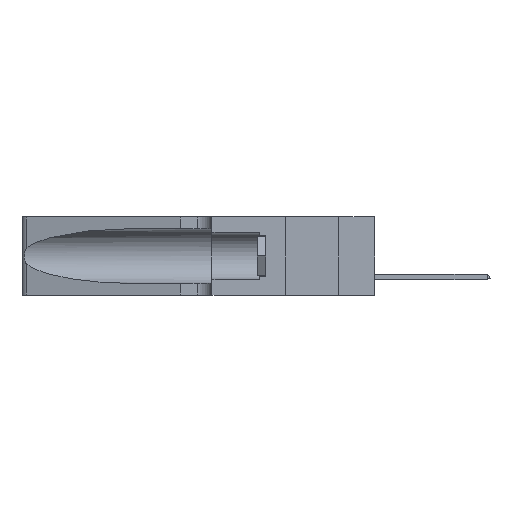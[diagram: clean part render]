
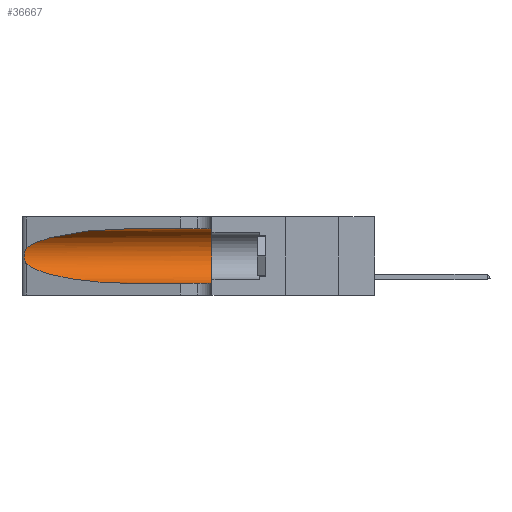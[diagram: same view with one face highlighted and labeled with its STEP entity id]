
A CAD part, left-side view. The second image highlights one B-rep face of the part: STEP entity #36667.
In plain terms, the highlighted cylindrical face has radius 3.308 mm (diameter 6.617 mm), a partial arc.
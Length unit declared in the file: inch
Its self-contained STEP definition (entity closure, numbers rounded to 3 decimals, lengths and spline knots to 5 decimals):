
#444 = CARTESIAN_POINT ( 'NONE',  ( 0.18966, 0.96281, 0.05475 ) ) ;
#1295 = LINE ( 'NONE', #36476, #23043 ) ;
#1427 = CYLINDRICAL_SURFACE ( 'NONE', #3161, 0.13025 ) ;
#3161 = AXIS2_PLACEMENT_3D ( 'NONE', #37629, #3948, #16302 ) ;
#3672 = ORIENTED_EDGE ( 'NONE', *, *, #19478, .F. ) ;
#3948 = DIRECTION ( 'NONE',  ( 0., -1., 0. ) ) ;
#4481 = CARTESIAN_POINT ( 'NONE',  ( 0.1305, 0.35, 0.31525 ) ) ;
#4510 = ORIENTED_EDGE ( 'NONE', *, *, #5658, .T. ) ;
#4600 = EDGE_CURVE ( 'NONE', #29638, #32882, #22584, .T. ) ;
#5658 = EDGE_CURVE ( 'NONE', #21468, #32882, #39531, .T. ) ;
#6064 = ORIENTED_EDGE ( 'NONE', *, *, #15649, .T. ) ;
#8571 = CARTESIAN_POINT ( 'NONE',  ( 0.2373, 1.15595, 0.28018 ) ) ;
#8985 = EDGE_LOOP ( 'NONE', ( #6064, #32623, #36070, #4510, #14835, #3672 ) ) ;
#9434 = CARTESIAN_POINT ( 'NONE',  ( 0.25787, 1.23484, 0.2124 ) ) ;
#9703 = CARTESIAN_POINT ( 'NONE',  ( 0.25639, 1.23184, 0.21858 ) ) ;
#12849 = CARTESIAN_POINT ( 'NONE',  ( 0.25789, 1.23486, 0.15765 ) ) ;
#14820 = VERTEX_POINT ( 'NONE', #22668 ) ;
#14829 = CARTESIAN_POINT ( 'NONE',  ( 0.25487, 1.22718, 0.22369 ) ) ;
#14835 = ORIENTED_EDGE ( 'NONE', *, *, #4600, .F. ) ;
#15131 = EDGE_CURVE ( 'NONE', #39350, #26571, #27689, .T. ) ;
#15649 = EDGE_CURVE ( 'NONE', #14820, #39350, #34888, .T. ) ;
#16302 = DIRECTION ( 'NONE',  ( 0., 0., -1. ) ) ;
#18497 = CARTESIAN_POINT ( 'NONE',  ( 0.26075, 1.23896, 0.178 ) ) ;
#18618 = CARTESIAN_POINT ( 'NONE',  ( 0.26018, 1.23835, 0.19895 ) ) ;
#18739 = CARTESIAN_POINT ( 'NONE',  ( 0.25487, 1.22718, 0.14631 ) ) ;
#18864 = CARTESIAN_POINT ( 'NONE',  ( 0.25639, 1.23186, 0.15144 ) ) ;
#18959 = CARTESIAN_POINT ( 'NONE',  ( 0.2373, 1.15595, 0.08982 ) ) ;
#19093 = CARTESIAN_POINT ( 'NONE',  ( 0.1305, 0.72297, 0.05475 ) ) ;
#19478 = EDGE_CURVE ( 'NONE', #14820, #29638, #1295, .T. ) ;
#20812 = CARTESIAN_POINT ( 'NONE',  ( 0.25487, 1.22718, 0.14631 ) ) ;
#20930 = DIRECTION ( 'NONE',  ( 0., -1., 0. ) ) ;
#21468 = VERTEX_POINT ( 'NONE', #21919 ) ;
#21919 = CARTESIAN_POINT ( 'NONE',  ( 0.1305, 0.72297, 0.05475 ) ) ;
#22584 = CIRCLE ( 'NONE', #39378, 0.13025 ) ;
#22668 = CARTESIAN_POINT ( 'NONE',  ( 0.1305, 0.72297, 0.31525 ) ) ;
#23043 = VECTOR ( 'NONE', #20930, 39.37008 ) ;
#23539 = VECTOR ( 'NONE', #24495, 39.37008 ) ;
#23828 = CARTESIAN_POINT ( 'NONE',  ( 0.1305, 1.61858, 0.05475 ) ) ;
#24495 = DIRECTION ( 'NONE',  ( 0., -1., 0. ) ) ;
#24626 = CARTESIAN_POINT ( 'NONE',  ( 0.1305, 0.35, 0.185 ) ) ;
#24688 = CARTESIAN_POINT ( 'NONE',  ( 0.25856, 1.23593, 0.16098 ) ) ;
#24704 =( BOUNDED_CURVE ( )  B_SPLINE_CURVE ( 3, ( #31270, #18959, #444, #19093 ),
 .UNSPECIFIED., .F., .F. ) 
 B_SPLINE_CURVE_WITH_KNOTS ( ( 4, 4 ),
 ( 3.44316, 4.71239 ),
 .UNSPECIFIED. ) 
 CURVE ( )  GEOMETRIC_REPRESENTATION_ITEM ( )  RATIONAL_B_SPLINE_CURVE ( ( 1., 0.87, 0.87, 1. ) ) 
 REPRESENTATION_ITEM ( '' )  );
#25073 = CARTESIAN_POINT ( 'NONE',  ( 0.25487, 1.22718, 0.22369 ) ) ;
#26571 = VERTEX_POINT ( 'NONE', #20812 ) ;
#27689 = B_SPLINE_CURVE_WITH_KNOTS ( 'NONE', 3,
 ( #25073, #28210, #9703, #9434, #34295, #18618, #31310, #18497, #34166, #24688, #12849, #18864, #27813, #18739 ),
 .UNSPECIFIED., .F., .F.,
 ( 4, 2, 2, 2, 2, 2, 4 ),
 ( 0., 0.00027, 0.00053, 0.00107, 0.0016, 0.00187, 0.00214 ),
 .UNSPECIFIED. ) ;
#27813 = CARTESIAN_POINT ( 'NONE',  ( 0.25555, 1.22993, 0.14849 ) ) ;
#27867 = DIRECTION ( 'NONE',  ( 0., 0., 1. ) ) ;
#28210 = CARTESIAN_POINT ( 'NONE',  ( 0.25555, 1.22994, 0.2215 ) ) ;
#29638 = VERTEX_POINT ( 'NONE', #4481 ) ;
#29960 = CARTESIAN_POINT ( 'NONE',  ( 0.18966, 0.96281, 0.31525 ) ) ;
#31270 = CARTESIAN_POINT ( 'NONE',  ( 0.25487, 1.22718, 0.14631 ) ) ;
#31310 = CARTESIAN_POINT ( 'NONE',  ( 0.26075, 1.23896, 0.19203 ) ) ;
#32623 = ORIENTED_EDGE ( 'NONE', *, *, #15131, .T. ) ;
#32882 = VERTEX_POINT ( 'NONE', #40065 ) ;
#33829 = DIRECTION ( 'NONE',  ( 0., 1., 0. ) ) ;
#34166 = CARTESIAN_POINT ( 'NONE',  ( 0.26017, 1.23833, 0.17102 ) ) ;
#34222 = EDGE_CURVE ( 'NONE', #26571, #21468, #24704, .T. ) ;
#34295 = CARTESIAN_POINT ( 'NONE',  ( 0.25854, 1.2359, 0.20912 ) ) ;
#34888 =( BOUNDED_CURVE ( )  B_SPLINE_CURVE ( 3, ( #39172, #29960, #8571, #14829 ),
 .UNSPECIFIED., .F., .F. ) 
 B_SPLINE_CURVE_WITH_KNOTS ( ( 4, 4 ),
 ( 1.5708, 2.84003 ),
 .UNSPECIFIED. ) 
 CURVE ( )  GEOMETRIC_REPRESENTATION_ITEM ( )  RATIONAL_B_SPLINE_CURVE ( ( 1., 0.87, 0.87, 1. ) ) 
 REPRESENTATION_ITEM ( '' )  );
#36023 = CARTESIAN_POINT ( 'NONE',  ( 0.25487, 1.22718, 0.22369 ) ) ;
#36070 = ORIENTED_EDGE ( 'NONE', *, *, #34222, .T. ) ;
#36476 = CARTESIAN_POINT ( 'NONE',  ( 0.1305, 1.61858, 0.31525 ) ) ;
#36667 = ADVANCED_FACE ( 'NONE', ( #36762 ), #1427, .F. ) ;
#36762 = FACE_OUTER_BOUND ( 'NONE', #8985, .T. ) ;
#37629 = CARTESIAN_POINT ( 'NONE',  ( 0.1305, 1.61858, 0.185 ) ) ;
#39172 = CARTESIAN_POINT ( 'NONE',  ( 0.1305, 0.72297, 0.31525 ) ) ;
#39350 = VERTEX_POINT ( 'NONE', #36023 ) ;
#39378 = AXIS2_PLACEMENT_3D ( 'NONE', #24626, #33829, #27867 ) ;
#39531 = LINE ( 'NONE', #23828, #23539 ) ;
#40065 = CARTESIAN_POINT ( 'NONE',  ( 0.1305, 0.35, 0.05475 ) ) ;
